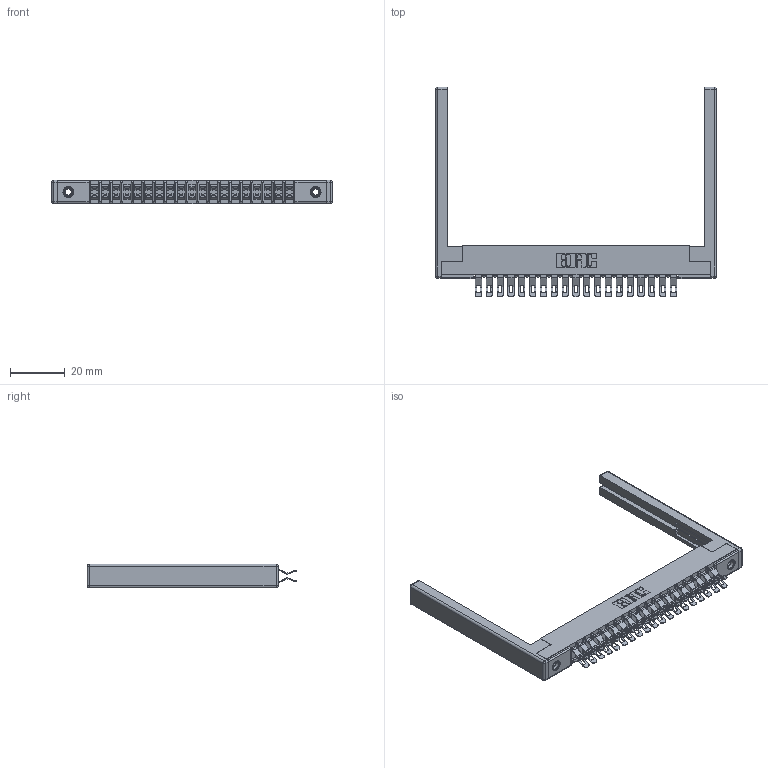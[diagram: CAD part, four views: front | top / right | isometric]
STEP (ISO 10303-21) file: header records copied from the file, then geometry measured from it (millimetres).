
FILE_DESCRIPTION (( 'STEP AP203' ), '1' );
FILE_NAME ('307-038-455-268.STEP', '2020-09-29T19:12:40', ( '' ), ( '' ), 'SwSTEP 2.0', 'SolidWorks 2020', '' );
FILE_SCHEMA (( 'CONFIG_CONTROL_DESIGN' ));
Length unit declared in the file: inch
Products named in the file (5): 307-290-001_555; 307-220-068; 345-250-001_345-250-001-102; 307-038-455-268; 307 Part_.156 Dia Mounting Holes
Assembly tree (43 placements, depth 2):
  307-038-455-268
    307 Part_.156 Dia Mounting Holes
    307-290-001_555  x38
    307-220-068  x2
    345-250-001_345-250-001-102  x2
Bounding box: 102.72 x 76.71 x 8.71 mm (x, y, z)
Volume: 11393.9 mm3; surface area: 16580.4 mm2
Topology: 43 solids, 43 shells, 2610 faces, 7591 edges, 4934 vertices
Faces by surface type: plane 1450, cylinder 1096, sphere 48, cone 12, torus 4
Entity records: 23028 total; most frequent: CARTESIAN_POINT 3756, ORIENTED_EDGE 3714, DIRECTION 3711, EDGE_CURVE 1857, VECTOR 1401, LINE 1401, VERTEX_POINT 1200, AXIS2_PLACEMENT_3D 1155
